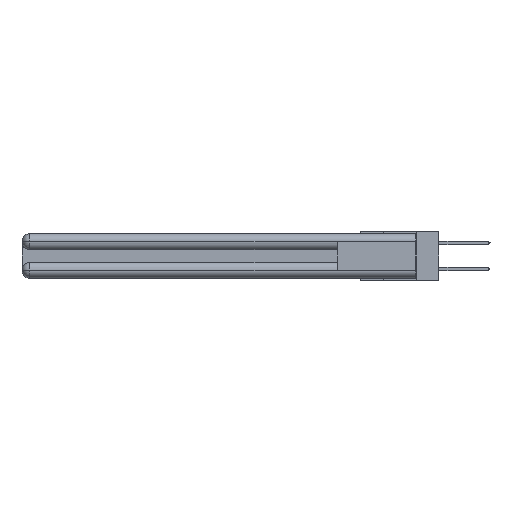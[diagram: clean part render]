
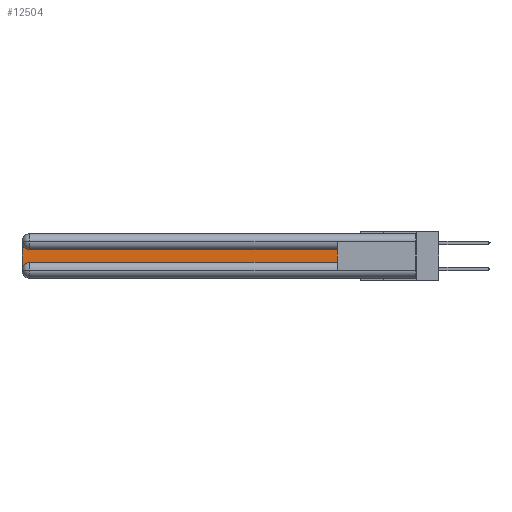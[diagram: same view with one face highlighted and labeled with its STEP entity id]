
A CAD part, left-side view. The second image highlights one B-rep face of the part: STEP entity #12504.
In plain terms, the highlighted planar face has unit normal (-1, 0, 0).
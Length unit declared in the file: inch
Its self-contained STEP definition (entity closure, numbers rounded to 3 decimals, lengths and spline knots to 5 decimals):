
#393 = EDGE_CURVE ( 'NONE', #25990, #21932, #16483, .T. ) ;
#664 = DIRECTION ( 'NONE',  ( 0., 0., -1. ) ) ;
#865 = CARTESIAN_POINT ( 'NONE',  ( 0.075, 0.6, -0.2175 ) ) ;
#1474 = DIRECTION ( 'NONE',  ( 0., 0., -1. ) ) ;
#1601 = CARTESIAN_POINT ( 'NONE',  ( 0.075, 0.6, -0.2175 ) ) ;
#1958 = CARTESIAN_POINT ( 'NONE',  ( 0.075, 0.6, -0.1225 ) ) ;
#2031 = ORIENTED_EDGE ( 'NONE', *, *, #25547, .T. ) ;
#3029 = EDGE_LOOP ( 'NONE', ( #17184, #3840, #26551, #3364, #2031, #4021 ) ) ;
#3364 = ORIENTED_EDGE ( 'NONE', *, *, #10177, .T. ) ;
#3764 = FACE_OUTER_BOUND ( 'NONE', #3029, .T. ) ;
#3840 = ORIENTED_EDGE ( 'NONE', *, *, #7869, .T. ) ;
#3970 = VECTOR ( 'NONE', #28447, 39.37008 ) ;
#4021 = ORIENTED_EDGE ( 'NONE', *, *, #18252, .T. ) ;
#4648 = CARTESIAN_POINT ( 'NONE',  ( 0.075, 0.6, -0.1225 ) ) ;
#4847 = AXIS2_PLACEMENT_3D ( 'NONE', #14291, #27881, #664 ) ;
#4970 = AXIS2_PLACEMENT_3D ( 'NONE', #14612, #27891, #7725 ) ;
#5702 = AXIS2_PLACEMENT_3D ( 'NONE', #12816, #28803, #1474 ) ;
#7042 = PLANE ( 'NONE',  #4847 ) ;
#7178 = CARTESIAN_POINT ( 'NONE',  ( 0.075, 3., -0.2175 ) ) ;
#7421 = LINE ( 'NONE', #1601, #8131 ) ;
#7725 = DIRECTION ( 'NONE',  ( 0., 0., -1. ) ) ;
#7869 = EDGE_CURVE ( 'NONE', #12465, #25990, #9352, .T. ) ;
#8131 = VECTOR ( 'NONE', #17714, 39.37008 ) ;
#8359 = LINE ( 'NONE', #865, #11192 ) ;
#9352 = CIRCLE ( 'NONE', #5702, 0.06 ) ;
#9693 = VECTOR ( 'NONE', #23092, 39.37008 ) ;
#10177 = EDGE_CURVE ( 'NONE', #21932, #17844, #22426, .T. ) ;
#11192 = VECTOR ( 'NONE', #21362, 39.37008 ) ;
#12005 = CARTESIAN_POINT ( 'NONE',  ( 0.075, 0.6, -0.2175 ) ) ;
#12465 = VERTEX_POINT ( 'NONE', #27467 ) ;
#12504 = ADVANCED_FACE ( 'NONE', ( #3764 ), #7042, .F. ) ;
#12816 = CARTESIAN_POINT ( 'NONE',  ( 0.075, 2.94, -0.0625 ) ) ;
#14291 = CARTESIAN_POINT ( 'NONE',  ( 0.075, 3., -0.1225 ) ) ;
#14612 = CARTESIAN_POINT ( 'NONE',  ( 0.075, 2.94, -0.2775 ) ) ;
#14946 = CARTESIAN_POINT ( 'NONE',  ( 0.075, 3., -0.0625 ) ) ;
#14980 = LINE ( 'NONE', #4648, #3970 ) ;
#16483 = LINE ( 'NONE', #7178, #9693 ) ;
#17184 = ORIENTED_EDGE ( 'NONE', *, *, #29528, .T. ) ;
#17714 = DIRECTION ( 'NONE',  ( 0., 0., 1. ) ) ;
#17844 = VERTEX_POINT ( 'NONE', #18226 ) ;
#18226 = CARTESIAN_POINT ( 'NONE',  ( 0.075, 2.94, -0.2175 ) ) ;
#18252 = EDGE_CURVE ( 'NONE', #21013, #18291, #7421, .T. ) ;
#18291 = VERTEX_POINT ( 'NONE', #1958 ) ;
#20885 = CARTESIAN_POINT ( 'NONE',  ( 0.075, 3., -0.2775 ) ) ;
#21013 = VERTEX_POINT ( 'NONE', #12005 ) ;
#21362 = DIRECTION ( 'NONE',  ( 0., -1., 0. ) ) ;
#21932 = VERTEX_POINT ( 'NONE', #20885 ) ;
#22426 = CIRCLE ( 'NONE', #4970, 0.06 ) ;
#23092 = DIRECTION ( 'NONE',  ( 0., 0., -1. ) ) ;
#25547 = EDGE_CURVE ( 'NONE', #17844, #21013, #8359, .T. ) ;
#25990 = VERTEX_POINT ( 'NONE', #14946 ) ;
#26551 = ORIENTED_EDGE ( 'NONE', *, *, #393, .T. ) ;
#27467 = CARTESIAN_POINT ( 'NONE',  ( 0.075, 2.94, -0.1225 ) ) ;
#27881 = DIRECTION ( 'NONE',  ( 1., 0., 0. ) ) ;
#27891 = DIRECTION ( 'NONE',  ( 1., 0., 0. ) ) ;
#28447 = DIRECTION ( 'NONE',  ( 0., 1., 0. ) ) ;
#28803 = DIRECTION ( 'NONE',  ( 1., 0., 0. ) ) ;
#29528 = EDGE_CURVE ( 'NONE', #18291, #12465, #14980, .T. ) ;
